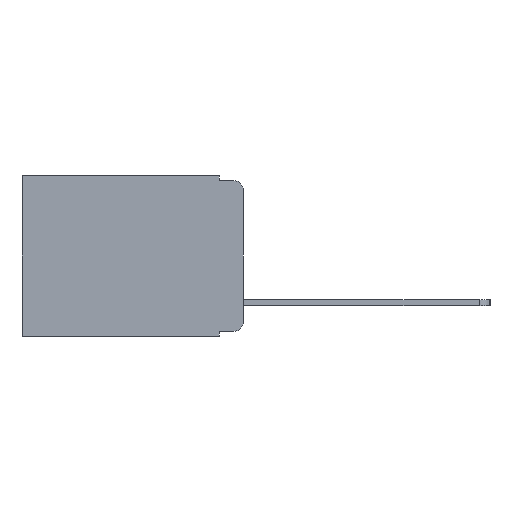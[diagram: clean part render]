
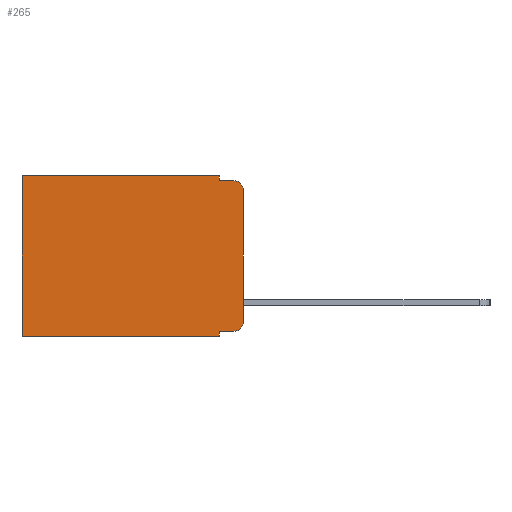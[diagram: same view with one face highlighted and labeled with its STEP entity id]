
A CAD part, left-side view. The second image highlights one B-rep face of the part: STEP entity #265.
In plain terms, the highlighted planar face has unit normal (-1, 0, 0).
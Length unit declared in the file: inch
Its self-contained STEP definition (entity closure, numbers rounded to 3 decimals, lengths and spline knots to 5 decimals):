
#7 = VERTEX_POINT ( 'NONE', #17585 ) ;
#265 = ADVANCED_FACE ( 'NONE', ( #17359 ), #5110, .F. ) ;
#1081 = DIRECTION ( 'NONE',  ( 0., 0., -1. ) ) ;
#1229 = EDGE_CURVE ( 'NONE', #15602, #18564, #7869, .T. ) ;
#1832 = EDGE_LOOP ( 'NONE', ( #10148, #18399, #6888, #15077, #17260, #6981, #6628, #15146, #4212, #15473 ) ) ;
#2063 = AXIS2_PLACEMENT_3D ( 'NONE', #12002, #9758, #9779 ) ;
#2334 = EDGE_CURVE ( 'NONE', #15091, #15602, #4712, .T. ) ;
#3096 = VECTOR ( 'NONE', #12809, 39.37008 ) ;
#3483 = LINE ( 'NONE', #15367, #14818 ) ;
#4212 = ORIENTED_EDGE ( 'NONE', *, *, #2334, .T. ) ;
#4493 = VERTEX_POINT ( 'NONE', #9034 ) ;
#4712 = LINE ( 'NONE', #13188, #15466 ) ;
#5008 = VERTEX_POINT ( 'NONE', #16460 ) ;
#5110 = PLANE ( 'NONE',  #2063 ) ;
#5155 = DIRECTION ( 'NONE',  ( 0., 1., 0. ) ) ;
#5368 = CARTESIAN_POINT ( 'NONE',  ( 0.298, 0.051, -0.333 ) ) ;
#5499 = EDGE_CURVE ( 'NONE', #15091, #4493, #15519, .T. ) ;
#6069 = CARTESIAN_POINT ( 'NONE',  ( 0.298, 0., -0.03 ) ) ;
#6071 = DIRECTION ( 'NONE',  ( 0., 0., -1. ) ) ;
#6408 = VECTOR ( 'NONE', #15623, 39.37008 ) ;
#6576 = CARTESIAN_POINT ( 'NONE',  ( 0.298, 0., -0.343 ) ) ;
#6628 = ORIENTED_EDGE ( 'NONE', *, *, #9029, .F. ) ;
#6888 = ORIENTED_EDGE ( 'NONE', *, *, #11471, .F. ) ;
#6981 = ORIENTED_EDGE ( 'NONE', *, *, #8530, .T. ) ;
#7684 = CARTESIAN_POINT ( 'NONE',  ( 0.298, 0.02, -0.313 ) ) ;
#7869 = CIRCLE ( 'NONE', #18391, 0.02 ) ;
#8169 = CARTESIAN_POINT ( 'NONE',  ( 0.298, 0.051, -0.01 ) ) ;
#8530 = EDGE_CURVE ( 'NONE', #5008, #17032, #14925, .T. ) ;
#8541 = VECTOR ( 'NONE', #19127, 39.37008 ) ;
#8789 = VERTEX_POINT ( 'NONE', #11986 ) ;
#8889 = DIRECTION ( 'NONE',  ( -1., 0., 0. ) ) ;
#9007 = LINE ( 'NONE', #17719, #8541 ) ;
#9029 = EDGE_CURVE ( 'NONE', #4493, #17032, #14908, .T. ) ;
#9034 = CARTESIAN_POINT ( 'NONE',  ( 0.298, 0.051, -0.343 ) ) ;
#9526 = CARTESIAN_POINT ( 'NONE',  ( 0.298, 0.473, -0.343 ) ) ;
#9758 = DIRECTION ( 'NONE',  ( 1., 0., 0. ) ) ;
#9779 = DIRECTION ( 'NONE',  ( 0., 0., -1. ) ) ;
#9916 = CARTESIAN_POINT ( 'NONE',  ( 0.298, 0.473, 0. ) ) ;
#10148 = ORIENTED_EDGE ( 'NONE', *, *, #16214, .F. ) ;
#10151 = VECTOR ( 'NONE', #12248, 39.37008 ) ;
#10408 = DIRECTION ( 'NONE',  ( 0., -1., 0. ) ) ;
#10513 = EDGE_CURVE ( 'NONE', #8789, #11349, #11066, .T. ) ;
#11066 = LINE ( 'NONE', #17909, #10151 ) ;
#11125 = VECTOR ( 'NONE', #13789, 39.37008 ) ;
#11296 = LINE ( 'NONE', #14200, #6408 ) ;
#11349 = VERTEX_POINT ( 'NONE', #8169 ) ;
#11471 = EDGE_CURVE ( 'NONE', #11349, #7, #11296, .T. ) ;
#11986 = CARTESIAN_POINT ( 'NONE',  ( 0.298, 0.051, 0. ) ) ;
#12002 = CARTESIAN_POINT ( 'NONE',  ( 0.298, 0., 0. ) ) ;
#12136 = EDGE_CURVE ( 'NONE', #8789, #5008, #3483, .T. ) ;
#12248 = DIRECTION ( 'NONE',  ( 0., 0., -1. ) ) ;
#12433 = EDGE_CURVE ( 'NONE', #16181, #7, #14126, .T. ) ;
#12809 = DIRECTION ( 'NONE',  ( 0., 0., -1. ) ) ;
#13188 = CARTESIAN_POINT ( 'NONE',  ( 0.298, 0.051, -0.333 ) ) ;
#13789 = DIRECTION ( 'NONE',  ( 0., 1., 0. ) ) ;
#13813 = CARTESIAN_POINT ( 'NONE',  ( 0.298, 0.02, -0.333 ) ) ;
#14126 = CIRCLE ( 'NONE', #15090, 0.02 ) ;
#14200 = CARTESIAN_POINT ( 'NONE',  ( 0.298, 0.051, -0.01 ) ) ;
#14818 = VECTOR ( 'NONE', #5155, 39.37008 ) ;
#14908 = LINE ( 'NONE', #6576, #11125 ) ;
#14925 = LINE ( 'NONE', #9916, #3096 ) ;
#15077 = ORIENTED_EDGE ( 'NONE', *, *, #10513, .F. ) ;
#15090 = AXIS2_PLACEMENT_3D ( 'NONE', #17482, #8889, #18905 ) ;
#15091 = VERTEX_POINT ( 'NONE', #5368 ) ;
#15146 = ORIENTED_EDGE ( 'NONE', *, *, #5499, .F. ) ;
#15367 = CARTESIAN_POINT ( 'NONE',  ( 0.298, 0., 0. ) ) ;
#15466 = VECTOR ( 'NONE', #10408, 39.37008 ) ;
#15473 = ORIENTED_EDGE ( 'NONE', *, *, #1229, .T. ) ;
#15519 = LINE ( 'NONE', #16020, #19292 ) ;
#15602 = VERTEX_POINT ( 'NONE', #13813 ) ;
#15623 = DIRECTION ( 'NONE',  ( 0., -1., 0. ) ) ;
#16020 = CARTESIAN_POINT ( 'NONE',  ( 0.298, 0.051, 0. ) ) ;
#16181 = VERTEX_POINT ( 'NONE', #6069 ) ;
#16214 = EDGE_CURVE ( 'NONE', #16181, #18564, #9007, .T. ) ;
#16460 = CARTESIAN_POINT ( 'NONE',  ( 0.298, 0.473, 0. ) ) ;
#16976 = CARTESIAN_POINT ( 'NONE',  ( 0.298, 0., -0.313 ) ) ;
#17032 = VERTEX_POINT ( 'NONE', #9526 ) ;
#17260 = ORIENTED_EDGE ( 'NONE', *, *, #12136, .T. ) ;
#17359 = FACE_OUTER_BOUND ( 'NONE', #1832, .T. ) ;
#17362 = DIRECTION ( 'NONE',  ( -1., 0., 0. ) ) ;
#17482 = CARTESIAN_POINT ( 'NONE',  ( 0.298, 0.02, -0.03 ) ) ;
#17585 = CARTESIAN_POINT ( 'NONE',  ( 0.298, 0.02, -0.01 ) ) ;
#17719 = CARTESIAN_POINT ( 'NONE',  ( 0.298, 0., 0. ) ) ;
#17909 = CARTESIAN_POINT ( 'NONE',  ( 0.298, 0.051, 0. ) ) ;
#18391 = AXIS2_PLACEMENT_3D ( 'NONE', #7684, #17362, #6071 ) ;
#18399 = ORIENTED_EDGE ( 'NONE', *, *, #12433, .T. ) ;
#18564 = VERTEX_POINT ( 'NONE', #16976 ) ;
#18905 = DIRECTION ( 'NONE',  ( 0., 0., -1. ) ) ;
#19127 = DIRECTION ( 'NONE',  ( 0., 0., -1. ) ) ;
#19292 = VECTOR ( 'NONE', #1081, 39.37008 ) ;
